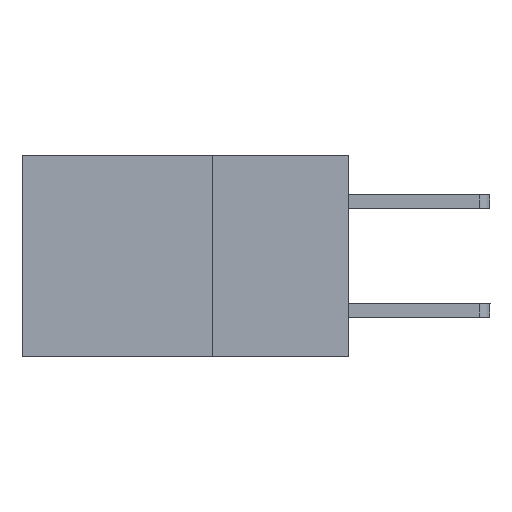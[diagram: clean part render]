
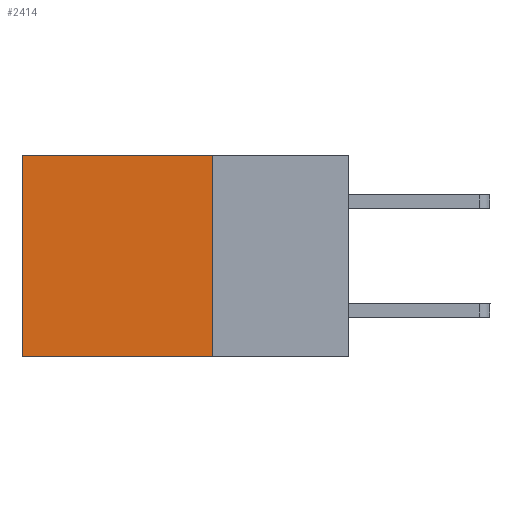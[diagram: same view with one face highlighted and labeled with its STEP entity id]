
A CAD part, left-side view. The second image highlights one B-rep face of the part: STEP entity #2414.
In plain terms, the highlighted planar face has unit normal (-1, 0, 0).
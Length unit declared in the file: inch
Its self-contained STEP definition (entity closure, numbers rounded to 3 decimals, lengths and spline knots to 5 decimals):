
#196 = VECTOR ( 'NONE', #10682, 39.37008 ) ;
#612 = LINE ( 'NONE', #2454, #9444 ) ;
#1192 = CARTESIAN_POINT ( 'NONE',  ( 0.298, 0.6, 0. ) ) ;
#1333 = DIRECTION ( 'NONE',  ( 0., 0., -1. ) ) ;
#1726 = VERTEX_POINT ( 'NONE', #6108 ) ;
#2078 = CARTESIAN_POINT ( 'NONE',  ( 0.298, 0.25, 0. ) ) ;
#2317 = VECTOR ( 'NONE', #9398, 39.37008 ) ;
#2414 = ADVANCED_FACE ( 'NONE', ( #3149 ), #5540, .F. ) ;
#2454 = CARTESIAN_POINT ( 'NONE',  ( 0.298, 0.25, -0.37 ) ) ;
#3149 = FACE_OUTER_BOUND ( 'NONE', #7552, .T. ) ;
#3238 = ORIENTED_EDGE ( 'NONE', *, *, #4411, .T. ) ;
#3975 = LINE ( 'NONE', #1192, #4514 ) ;
#4411 = EDGE_CURVE ( 'NONE', #10251, #1726, #3975, .T. ) ;
#4413 = DIRECTION ( 'NONE',  ( 0., 1., 0. ) ) ;
#4514 = VECTOR ( 'NONE', #9724, 39.37008 ) ;
#4622 = ORIENTED_EDGE ( 'NONE', *, *, #9786, .F. ) ;
#4727 = LINE ( 'NONE', #2078, #196 ) ;
#5540 = PLANE ( 'NONE',  #8260 ) ;
#6108 = CARTESIAN_POINT ( 'NONE',  ( 0.298, 0.6, -0.37 ) ) ;
#6222 = ORIENTED_EDGE ( 'NONE', *, *, #10464, .T. ) ;
#6495 = CARTESIAN_POINT ( 'NONE',  ( 0.298, 0.25, 0. ) ) ;
#6727 = VERTEX_POINT ( 'NONE', #9874 ) ;
#6917 = CARTESIAN_POINT ( 'NONE',  ( 0.298, 0.6, 0. ) ) ;
#7019 = EDGE_CURVE ( 'NONE', #8929, #6727, #10215, .T. ) ;
#7301 = CARTESIAN_POINT ( 'NONE',  ( 0.298, 0.25, 0. ) ) ;
#7552 = EDGE_LOOP ( 'NONE', ( #3238, #4622, #9745, #6222 ) ) ;
#8260 = AXIS2_PLACEMENT_3D ( 'NONE', #6495, #10851, #1333 ) ;
#8929 = VERTEX_POINT ( 'NONE', #7301 ) ;
#9363 = CARTESIAN_POINT ( 'NONE',  ( 0.298, 0.25, 0. ) ) ;
#9398 = DIRECTION ( 'NONE',  ( 0., 0., -1. ) ) ;
#9444 = VECTOR ( 'NONE', #4413, 39.37008 ) ;
#9724 = DIRECTION ( 'NONE',  ( 0., 0., -1. ) ) ;
#9745 = ORIENTED_EDGE ( 'NONE', *, *, #7019, .F. ) ;
#9786 = EDGE_CURVE ( 'NONE', #6727, #1726, #612, .T. ) ;
#9874 = CARTESIAN_POINT ( 'NONE',  ( 0.298, 0.25, -0.37 ) ) ;
#10215 = LINE ( 'NONE', #9363, #2317 ) ;
#10251 = VERTEX_POINT ( 'NONE', #6917 ) ;
#10464 = EDGE_CURVE ( 'NONE', #8929, #10251, #4727, .T. ) ;
#10682 = DIRECTION ( 'NONE',  ( 0., 1., 0. ) ) ;
#10851 = DIRECTION ( 'NONE',  ( 1., 0., 0. ) ) ;
